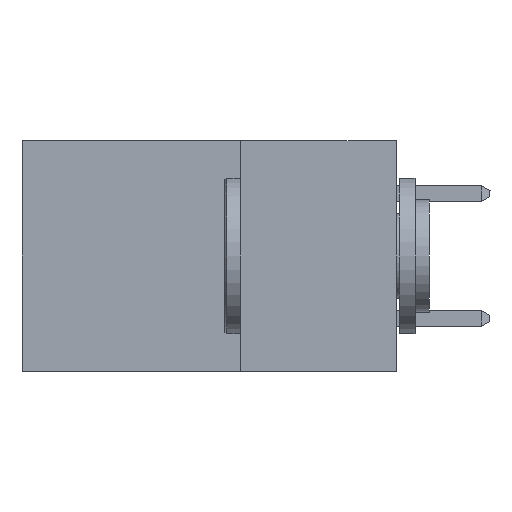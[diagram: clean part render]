
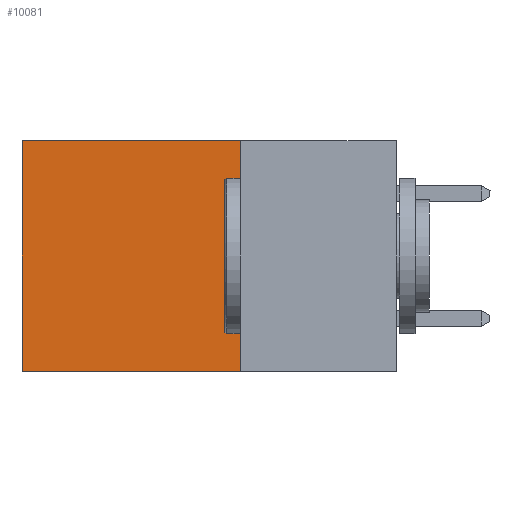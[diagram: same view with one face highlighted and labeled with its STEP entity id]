
A CAD part, left-side view. The second image highlights one B-rep face of the part: STEP entity #10081.
In plain terms, the highlighted planar face has unit normal (-1, 0, 0).
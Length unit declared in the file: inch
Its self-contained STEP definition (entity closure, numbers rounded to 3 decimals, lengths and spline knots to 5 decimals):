
#271 = VERTEX_POINT ( 'NONE', #1460 ) ;
#1460 = CARTESIAN_POINT ( 'NONE',  ( 0.298, 0.25, -0.37 ) ) ;
#1527 = EDGE_CURVE ( 'NONE', #271, #9470, #2535, .T. ) ;
#2535 = LINE ( 'NONE', #10264, #9165 ) ;
#4178 = VERTEX_POINT ( 'NONE', #4388 ) ;
#4388 = CARTESIAN_POINT ( 'NONE',  ( 0.298, 0.25, 0. ) ) ;
#4642 = CARTESIAN_POINT ( 'NONE',  ( 0.298, 0.6, -0.37 ) ) ;
#4944 = VECTOR ( 'NONE', #12079, 39.37008 ) ;
#5715 = FACE_OUTER_BOUND ( 'NONE', #5877, .T. ) ;
#5877 = EDGE_LOOP ( 'NONE', ( #7681, #14073, #8052, #8842 ) ) ;
#6203 = DIRECTION ( 'NONE',  ( 0., 0., -1. ) ) ;
#7160 = DIRECTION ( 'NONE',  ( 1., 0., 0. ) ) ;
#7369 = EDGE_CURVE ( 'NONE', #11922, #9470, #15760, .T. ) ;
#7681 = ORIENTED_EDGE ( 'NONE', *, *, #7369, .T. ) ;
#8052 = ORIENTED_EDGE ( 'NONE', *, *, #10857, .F. ) ;
#8122 = VECTOR ( 'NONE', #15266, 39.37008 ) ;
#8349 = CARTESIAN_POINT ( 'NONE',  ( 0.298, 0.25, 0. ) ) ;
#8689 = LINE ( 'NONE', #9889, #15046 ) ;
#8842 = ORIENTED_EDGE ( 'NONE', *, *, #10150, .T. ) ;
#9165 = VECTOR ( 'NONE', #10894, 39.37008 ) ;
#9278 = CARTESIAN_POINT ( 'NONE',  ( 0.298, 0.6, 0. ) ) ;
#9470 = VERTEX_POINT ( 'NONE', #4642 ) ;
#9889 = CARTESIAN_POINT ( 'NONE',  ( 0.298, 0.25, 0. ) ) ;
#10081 = ADVANCED_FACE ( 'NONE', ( #5715 ), #15495, .F. ) ;
#10150 = EDGE_CURVE ( 'NONE', #4178, #11922, #14243, .T. ) ;
#10264 = CARTESIAN_POINT ( 'NONE',  ( 0.298, 0.25, -0.37 ) ) ;
#10857 = EDGE_CURVE ( 'NONE', #4178, #271, #8689, .T. ) ;
#10894 = DIRECTION ( 'NONE',  ( 0., 1., 0. ) ) ;
#11922 = VERTEX_POINT ( 'NONE', #9278 ) ;
#12079 = DIRECTION ( 'NONE',  ( 0., 1., 0. ) ) ;
#12198 = AXIS2_PLACEMENT_3D ( 'NONE', #8349, #7160, #15541 ) ;
#14073 = ORIENTED_EDGE ( 'NONE', *, *, #1527, .F. ) ;
#14243 = LINE ( 'NONE', #15646, #4944 ) ;
#15046 = VECTOR ( 'NONE', #6203, 39.37008 ) ;
#15266 = DIRECTION ( 'NONE',  ( 0., 0., -1. ) ) ;
#15426 = CARTESIAN_POINT ( 'NONE',  ( 0.298, 0.6, 0. ) ) ;
#15495 = PLANE ( 'NONE',  #12198 ) ;
#15541 = DIRECTION ( 'NONE',  ( 0., 0., -1. ) ) ;
#15646 = CARTESIAN_POINT ( 'NONE',  ( 0.298, 0.25, 0. ) ) ;
#15760 = LINE ( 'NONE', #15426, #8122 ) ;
